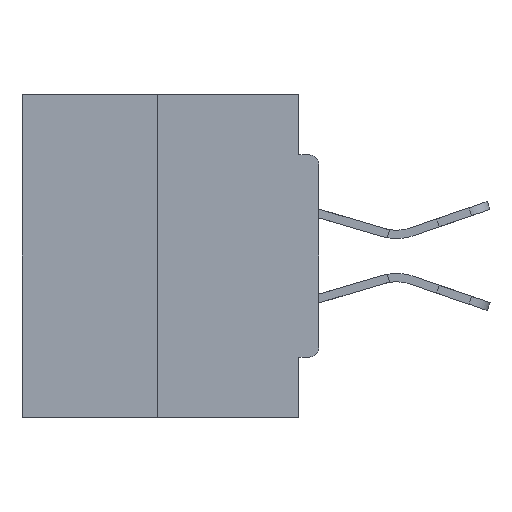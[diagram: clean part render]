
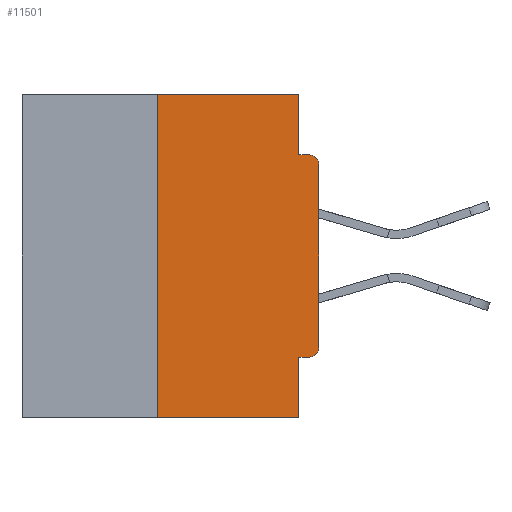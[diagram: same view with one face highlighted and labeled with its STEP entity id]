
A CAD part, left-side view. The second image highlights one B-rep face of the part: STEP entity #11501.
In plain terms, the highlighted planar face has unit normal (-1, 0, 0).
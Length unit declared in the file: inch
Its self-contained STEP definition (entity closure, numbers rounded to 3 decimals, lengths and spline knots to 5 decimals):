
#805 = VECTOR ( 'NONE', #34170, 39.37008 ) ;
#1176 = LINE ( 'NONE', #3773, #1638 ) ;
#1315 = DIRECTION ( 'NONE',  ( 1., 0., 0. ) ) ;
#1638 = VECTOR ( 'NONE', #18359, 39.37008 ) ;
#1773 = AXIS2_PLACEMENT_3D ( 'NONE', #30950, #19183, #21798 ) ;
#1952 = VERTEX_POINT ( 'NONE', #7757 ) ;
#2975 = AXIS2_PLACEMENT_3D ( 'NONE', #33845, #8221, #31225 ) ;
#3189 = CARTESIAN_POINT ( 'NONE',  ( 0., 0.031, -0.5 ) ) ;
#3773 = CARTESIAN_POINT ( 'NONE',  ( 0., 0., -0.4065 ) ) ;
#3806 = VECTOR ( 'NONE', #30688, 39.37008 ) ;
#4060 = ORIENTED_EDGE ( 'NONE', *, *, #27311, .F. ) ;
#4769 = ORIENTED_EDGE ( 'NONE', *, *, #16708, .F. ) ;
#5236 = ORIENTED_EDGE ( 'NONE', *, *, #17102, .T. ) ;
#6135 = CARTESIAN_POINT ( 'NONE',  ( 0., 0.46, 0. ) ) ;
#6322 = FACE_OUTER_BOUND ( 'NONE', #35675, .T. ) ;
#6791 = ORIENTED_EDGE ( 'NONE', *, *, #16631, .T. ) ;
#7757 = CARTESIAN_POINT ( 'NONE',  ( 0., 0.015, -0.4065 ) ) ;
#7915 = ORIENTED_EDGE ( 'NONE', *, *, #17776, .T. ) ;
#8056 = LINE ( 'NONE', #34237, #34405 ) ;
#8221 = DIRECTION ( 'NONE',  ( -1., 0., 0. ) ) ;
#8356 = EDGE_CURVE ( 'NONE', #14444, #24335, #33618, .T. ) ;
#8362 = CARTESIAN_POINT ( 'NONE',  ( 0., 0.031, -0.5 ) ) ;
#8424 = LINE ( 'NONE', #19828, #3806 ) ;
#8783 = CARTESIAN_POINT ( 'NONE',  ( 0., 0.015, -0.0935 ) ) ;
#9085 = CARTESIAN_POINT ( 'NONE',  ( 0., 0.031, -0.0935 ) ) ;
#9934 = VERTEX_POINT ( 'NONE', #12836 ) ;
#10044 = CARTESIAN_POINT ( 'NONE',  ( 0., 0., -0.3915 ) ) ;
#10463 = EDGE_CURVE ( 'NONE', #32165, #24335, #15503, .T. ) ;
#11501 = ADVANCED_FACE ( 'NONE', ( #6322 ), #14956, .F. ) ;
#12834 = DIRECTION ( 'NONE',  ( 0., 0., 1. ) ) ;
#12836 = CARTESIAN_POINT ( 'NONE',  ( 0., 0., -0.1085 ) ) ;
#12970 = VERTEX_POINT ( 'NONE', #9085 ) ;
#13381 = ORIENTED_EDGE ( 'NONE', *, *, #21858, .F. ) ;
#13458 = EDGE_CURVE ( 'NONE', #12970, #27609, #14635, .T. ) ;
#14156 = CARTESIAN_POINT ( 'NONE',  ( 0., 0.031, -0.4065 ) ) ;
#14444 = VERTEX_POINT ( 'NONE', #14156 ) ;
#14635 = LINE ( 'NONE', #22510, #30311 ) ;
#14956 = PLANE ( 'NONE',  #34344 ) ;
#14994 = VECTOR ( 'NONE', #12834, 39.37008 ) ;
#15503 = LINE ( 'NONE', #27074, #34657 ) ;
#16015 = LINE ( 'NONE', #18072, #14994 ) ;
#16416 = ORIENTED_EDGE ( 'NONE', *, *, #10463, .T. ) ;
#16631 = EDGE_CURVE ( 'NONE', #9934, #27609, #26837, .T. ) ;
#16708 = EDGE_CURVE ( 'NONE', #32165, #18586, #26255, .T. ) ;
#16876 = ORIENTED_EDGE ( 'NONE', *, *, #13458, .F. ) ;
#17102 = EDGE_CURVE ( 'NONE', #1952, #20757, #34023, .T. ) ;
#17153 = VERTEX_POINT ( 'NONE', #17749 ) ;
#17749 = CARTESIAN_POINT ( 'NONE',  ( 0., 0.031, 0. ) ) ;
#17776 = EDGE_CURVE ( 'NONE', #20757, #9934, #16015, .T. ) ;
#17869 = VECTOR ( 'NONE', #34676, 39.37008 ) ;
#18072 = CARTESIAN_POINT ( 'NONE',  ( 0., 0., 0. ) ) ;
#18359 = DIRECTION ( 'NONE',  ( 0., 1., 0. ) ) ;
#18586 = VERTEX_POINT ( 'NONE', #32731 ) ;
#19183 = DIRECTION ( 'NONE',  ( -1., 0., 0. ) ) ;
#19828 = CARTESIAN_POINT ( 'NONE',  ( 0., 0.031, 0. ) ) ;
#19885 = DIRECTION ( 'NONE',  ( 0., -1., 0. ) ) ;
#20757 = VERTEX_POINT ( 'NONE', #10044 ) ;
#21094 = CARTESIAN_POINT ( 'NONE',  ( 0., 0.25, -0.5 ) ) ;
#21470 = DIRECTION ( 'NONE',  ( 0., -1., 0. ) ) ;
#21798 = DIRECTION ( 'NONE',  ( 0., 0., -1. ) ) ;
#21858 = EDGE_CURVE ( 'NONE', #18586, #17153, #8056, .T. ) ;
#22510 = CARTESIAN_POINT ( 'NONE',  ( 0., 0., -0.0935 ) ) ;
#24335 = VERTEX_POINT ( 'NONE', #3189 ) ;
#25105 = ORIENTED_EDGE ( 'NONE', *, *, #35725, .F. ) ;
#26255 = LINE ( 'NONE', #31496, #17869 ) ;
#26837 = CIRCLE ( 'NONE', #1773, 0.015 ) ;
#27073 = ORIENTED_EDGE ( 'NONE', *, *, #8356, .F. ) ;
#27074 = CARTESIAN_POINT ( 'NONE',  ( 0., 0.46, -0.5 ) ) ;
#27311 = EDGE_CURVE ( 'NONE', #1952, #14444, #1176, .T. ) ;
#27609 = VERTEX_POINT ( 'NONE', #8783 ) ;
#28968 = DIRECTION ( 'NONE',  ( 0., 0., -1. ) ) ;
#30311 = VECTOR ( 'NONE', #19885, 39.37008 ) ;
#30688 = DIRECTION ( 'NONE',  ( 0., 0., -1. ) ) ;
#30950 = CARTESIAN_POINT ( 'NONE',  ( 0., 0.015, -0.1085 ) ) ;
#31225 = DIRECTION ( 'NONE',  ( 0., 0., -1. ) ) ;
#31496 = CARTESIAN_POINT ( 'NONE',  ( 0., 0.25, 0. ) ) ;
#32165 = VERTEX_POINT ( 'NONE', #21094 ) ;
#32731 = CARTESIAN_POINT ( 'NONE',  ( 0., 0.25, 0. ) ) ;
#33618 = LINE ( 'NONE', #8362, #805 ) ;
#33845 = CARTESIAN_POINT ( 'NONE',  ( 0., 0.015, -0.3915 ) ) ;
#33874 = DIRECTION ( 'NONE',  ( 0., -1., 0. ) ) ;
#34023 = CIRCLE ( 'NONE', #2975, 0.015 ) ;
#34170 = DIRECTION ( 'NONE',  ( 0., 0., -1. ) ) ;
#34237 = CARTESIAN_POINT ( 'NONE',  ( 0., 0.46, 0. ) ) ;
#34344 = AXIS2_PLACEMENT_3D ( 'NONE', #6135, #1315, #28968 ) ;
#34405 = VECTOR ( 'NONE', #33874, 39.37008 ) ;
#34657 = VECTOR ( 'NONE', #21470, 39.37008 ) ;
#34676 = DIRECTION ( 'NONE',  ( 0., 0., 1. ) ) ;
#35675 = EDGE_LOOP ( 'NONE', ( #13381, #4769, #16416, #27073, #4060, #5236, #7915, #6791, #16876, #25105 ) ) ;
#35725 = EDGE_CURVE ( 'NONE', #17153, #12970, #8424, .T. ) ;
